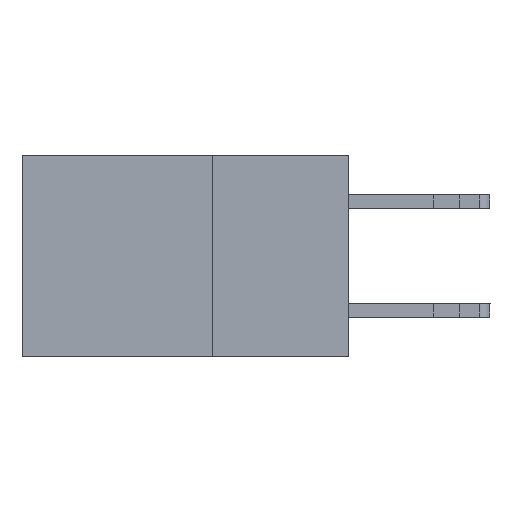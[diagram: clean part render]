
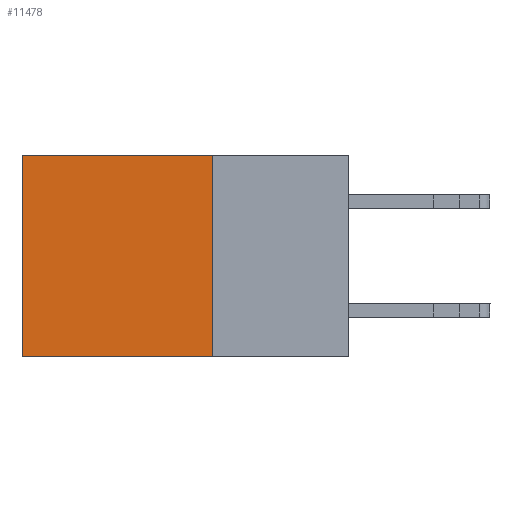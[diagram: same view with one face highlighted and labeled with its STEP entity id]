
A CAD part, left-side view. The second image highlights one B-rep face of the part: STEP entity #11478.
In plain terms, the highlighted planar face has unit normal (-1, 0, 0).
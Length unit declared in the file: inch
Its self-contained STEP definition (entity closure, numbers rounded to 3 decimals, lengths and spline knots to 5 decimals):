
#635 = FACE_OUTER_BOUND ( 'NONE', #8731, .T. ) ;
#1018 = VERTEX_POINT ( 'NONE', #7441 ) ;
#1044 = EDGE_CURVE ( 'NONE', #2054, #7128, #3614, .T. ) ;
#1527 = CARTESIAN_POINT ( 'NONE',  ( 0.2615, 0.25, -0.37 ) ) ;
#1622 = ORIENTED_EDGE ( 'NONE', *, *, #4813, .T. ) ;
#1647 = CARTESIAN_POINT ( 'NONE',  ( 0.2615, 0.25, -0.37 ) ) ;
#2054 = VERTEX_POINT ( 'NONE', #10488 ) ;
#2066 = ORIENTED_EDGE ( 'NONE', *, *, #1044, .F. ) ;
#2685 = EDGE_CURVE ( 'NONE', #1018, #10303, #5777, .T. ) ;
#2867 = DIRECTION ( 'NONE',  ( 0., 0., -1. ) ) ;
#2965 = DIRECTION ( 'NONE',  ( 1., 0., 0. ) ) ;
#3026 = DIRECTION ( 'NONE',  ( 0., 1., 0. ) ) ;
#3537 = LINE ( 'NONE', #10124, #8206 ) ;
#3614 = LINE ( 'NONE', #1527, #3898 ) ;
#3709 = LINE ( 'NONE', #6274, #6596 ) ;
#3715 = VECTOR ( 'NONE', #4113, 39.37008 ) ;
#3840 = PLANE ( 'NONE',  #5850 ) ;
#3898 = VECTOR ( 'NONE', #2867, 39.37008 ) ;
#4113 = DIRECTION ( 'NONE',  ( 0., 0., -1. ) ) ;
#4595 = ORIENTED_EDGE ( 'NONE', *, *, #7219, .F. ) ;
#4813 = EDGE_CURVE ( 'NONE', #2054, #1018, #3537, .T. ) ;
#5777 = LINE ( 'NONE', #9384, #3715 ) ;
#5850 = AXIS2_PLACEMENT_3D ( 'NONE', #8257, #2965, #9152 ) ;
#6193 = ORIENTED_EDGE ( 'NONE', *, *, #2685, .T. ) ;
#6274 = CARTESIAN_POINT ( 'NONE',  ( 0.2615, 0.25, -0.37 ) ) ;
#6596 = VECTOR ( 'NONE', #9795, 39.37008 ) ;
#7128 = VERTEX_POINT ( 'NONE', #1647 ) ;
#7219 = EDGE_CURVE ( 'NONE', #7128, #10303, #3709, .T. ) ;
#7441 = CARTESIAN_POINT ( 'NONE',  ( 0.2615, 0.6, 0. ) ) ;
#8206 = VECTOR ( 'NONE', #3026, 39.37008 ) ;
#8257 = CARTESIAN_POINT ( 'NONE',  ( 0.2615, 0.25, -0.37 ) ) ;
#8731 = EDGE_LOOP ( 'NONE', ( #6193, #4595, #2066, #1622 ) ) ;
#9152 = DIRECTION ( 'NONE',  ( 0., 0., -1. ) ) ;
#9384 = CARTESIAN_POINT ( 'NONE',  ( 0.2615, 0.6, -0.37 ) ) ;
#9795 = DIRECTION ( 'NONE',  ( 0., 1., 0. ) ) ;
#10124 = CARTESIAN_POINT ( 'NONE',  ( 0.2615, 0.25, 0. ) ) ;
#10303 = VERTEX_POINT ( 'NONE', #10562 ) ;
#10488 = CARTESIAN_POINT ( 'NONE',  ( 0.2615, 0.25, 0. ) ) ;
#10562 = CARTESIAN_POINT ( 'NONE',  ( 0.2615, 0.6, -0.37 ) ) ;
#11478 = ADVANCED_FACE ( 'NONE', ( #635 ), #3840, .F. ) ;
